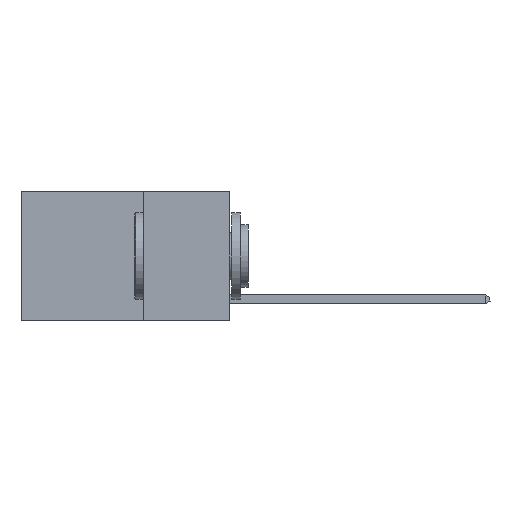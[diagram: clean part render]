
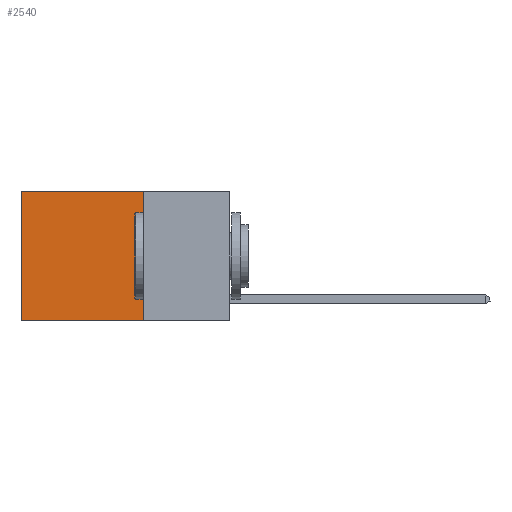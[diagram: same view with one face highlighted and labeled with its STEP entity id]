
A CAD part, left-side view. The second image highlights one B-rep face of the part: STEP entity #2540.
In plain terms, the highlighted planar face has unit normal (-1, 0, 0).
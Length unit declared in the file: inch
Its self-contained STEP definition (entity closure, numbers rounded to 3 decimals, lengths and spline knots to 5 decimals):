
#102 = ORIENTED_EDGE ( 'NONE', *, *, #21902, .T. ) ;
#264 = LINE ( 'NONE', #1859, #21513 ) ;
#329 = DIRECTION ( 'NONE',  ( 0., 0., -1. ) ) ;
#393 = ORIENTED_EDGE ( 'NONE', *, *, #21646, .T. ) ;
#672 = FACE_OUTER_BOUND ( 'NONE', #19231, .T. ) ;
#875 = CARTESIAN_POINT ( 'NONE',  ( 0.2625, 0.25, 0. ) ) ;
#1584 = CARTESIAN_POINT ( 'NONE',  ( 0.2625, 0.25, 0. ) ) ;
#1859 = CARTESIAN_POINT ( 'NONE',  ( 0.2625, 0.25, 0. ) ) ;
#2540 = ADVANCED_FACE ( 'NONE', ( #672 ), #5689, .F. ) ;
#2942 = DIRECTION ( 'NONE',  ( 0., 1., 0. ) ) ;
#3625 = DIRECTION ( 'NONE',  ( 0., 0., -1. ) ) ;
#5689 = PLANE ( 'NONE',  #8015 ) ;
#5698 = VERTEX_POINT ( 'NONE', #11246 ) ;
#7184 = DIRECTION ( 'NONE',  ( 0., 0., -1. ) ) ;
#7421 = CARTESIAN_POINT ( 'NONE',  ( 0.2625, 0.6, 0. ) ) ;
#7809 = CARTESIAN_POINT ( 'NONE',  ( 0.2625, 0.6, 0. ) ) ;
#8015 = AXIS2_PLACEMENT_3D ( 'NONE', #12706, #9228, #329 ) ;
#9197 = ORIENTED_EDGE ( 'NONE', *, *, #19323, .F. ) ;
#9228 = DIRECTION ( 'NONE',  ( 1., 0., 0. ) ) ;
#9959 = VERTEX_POINT ( 'NONE', #1584 ) ;
#11246 = CARTESIAN_POINT ( 'NONE',  ( 0.2625, 0.6, -0.37 ) ) ;
#11427 = VERTEX_POINT ( 'NONE', #7421 ) ;
#11574 = CARTESIAN_POINT ( 'NONE',  ( 0.2625, 0.25, -0.37 ) ) ;
#11789 = LINE ( 'NONE', #875, #20630 ) ;
#12706 = CARTESIAN_POINT ( 'NONE',  ( 0.2625, 0.25, 0. ) ) ;
#13413 = CARTESIAN_POINT ( 'NONE',  ( 0.2625, 0.25, -0.37 ) ) ;
#14135 = LINE ( 'NONE', #11574, #17695 ) ;
#15720 = EDGE_CURVE ( 'NONE', #9959, #21401, #264, .T. ) ;
#16878 = DIRECTION ( 'NONE',  ( 0., 1., 0. ) ) ;
#17695 = VECTOR ( 'NONE', #2942, 39.37008 ) ;
#19231 = EDGE_LOOP ( 'NONE', ( #393, #9197, #20598, #102 ) ) ;
#19323 = EDGE_CURVE ( 'NONE', #21401, #5698, #14135, .T. ) ;
#20064 = VECTOR ( 'NONE', #7184, 39.37008 ) ;
#20598 = ORIENTED_EDGE ( 'NONE', *, *, #15720, .F. ) ;
#20630 = VECTOR ( 'NONE', #16878, 39.37008 ) ;
#21401 = VERTEX_POINT ( 'NONE', #13413 ) ;
#21513 = VECTOR ( 'NONE', #3625, 39.37008 ) ;
#21646 = EDGE_CURVE ( 'NONE', #11427, #5698, #21733, .T. ) ;
#21733 = LINE ( 'NONE', #7809, #20064 ) ;
#21902 = EDGE_CURVE ( 'NONE', #9959, #11427, #11789, .T. ) ;
